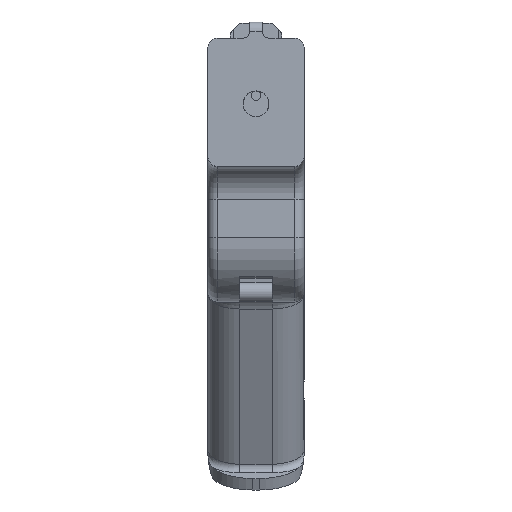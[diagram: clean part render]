
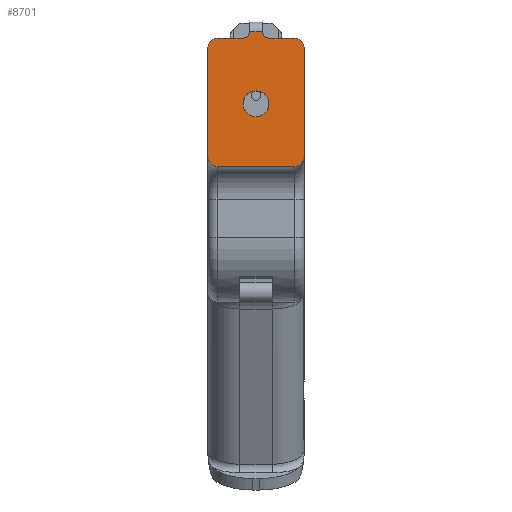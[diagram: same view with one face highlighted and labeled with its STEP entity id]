
A CAD part, top view. The second image highlights one B-rep face of the part: STEP entity #8701.
In plain terms, the highlighted planar face has unit normal (0, 0, 1).
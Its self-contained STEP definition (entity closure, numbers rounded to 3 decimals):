
#580=CARTESIAN_POINT('',(15.0,-3.,-20.));
#581=VERTEX_POINT('',#580);
#588=CARTESIAN_POINT('',(15.0,-37.,-20.));
#589=VERTEX_POINT('',#588);
#590=CARTESIAN_POINT('',(15.0,-3.,-20.));
#591=DIRECTION('',(0.0,-1.0,0.0));
#592=VECTOR('',#591,34.);
#593=LINE('',#590,#592);
#594=EDGE_CURVE('',#581,#589,#593,.T.);
#2318=CARTESIAN_POINT('',(-12.0,0.,-20.));
#2319=VERTEX_POINT('',#2318);
#2326=CARTESIAN_POINT('',(-4.0,0.,-20.));
#2327=VERTEX_POINT('',#2326);
#2328=CARTESIAN_POINT('',(-12.0,0.,-20.));
#2329=DIRECTION('',(1.0,0.0,0.0));
#2330=VECTOR('',#2329,8.0);
#2331=LINE('',#2328,#2330);
#2332=EDGE_CURVE('',#2319,#2327,#2331,.T.);
#2350=CARTESIAN_POINT('',(4.0,0.,-20.));
#2351=VERTEX_POINT('',#2350);
#2358=CARTESIAN_POINT('',(12.0,0.,-20.));
#2359=VERTEX_POINT('',#2358);
#2360=CARTESIAN_POINT('',(4.0,0.,-20.));
#2361=DIRECTION('',(1.0,0.0,0.0));
#2362=VECTOR('',#2361,8.0);
#2363=LINE('',#2360,#2362);
#2364=EDGE_CURVE('',#2351,#2359,#2363,.T.);
#8549=CARTESIAN_POINT('',(2.0,2.,-20.));
#8550=VERTEX_POINT('',#8549);
#8568=CARTESIAN_POINT('',(-2.0,2.,-20.));
#8569=VERTEX_POINT('',#8568);
#8577=CARTESIAN_POINT('',(-2.0,2.,-20.));
#8578=DIRECTION('',(1.0,0.0,0.0));
#8579=VECTOR('',#8578,4.0);
#8580=LINE('',#8577,#8579);
#8581=EDGE_CURVE('',#8569,#8550,#8580,.T.);
#8617=CARTESIAN_POINT('',(0.0,43.,-20.));
#8618=DIRECTION('',(0.0,0.0,-1.0));
#8619=DIRECTION('',(-1.0,0.0,0.0));
#8620=AXIS2_PLACEMENT_3D('',#8617,#8618,#8619);
#8621=PLANE('',#8620);
#8622=ORIENTED_EDGE('',*,*,#8581,.F.);
#8623=CARTESIAN_POINT('',(-4.0,2.,-20.));
#8624=DIRECTION('',(0.0,0.0,1.0));
#8625=DIRECTION('',(0.707,-0.707,0.0));
#8626=AXIS2_PLACEMENT_3D('',#8623,#8624,#8625);
#8627=CIRCLE('',#8626,2.0);
#8628=EDGE_CURVE('',#2327,#8569,#8627,.T.);
#8629=ORIENTED_EDGE('',*,*,#8628,.F.);
#8630=ORIENTED_EDGE('',*,*,#2332,.F.);
#8631=CARTESIAN_POINT('',(-15.0,-3.,-20.));
#8632=VERTEX_POINT('',#8631);
#8633=CARTESIAN_POINT('',(-12.0,-3.,-20.));
#8634=DIRECTION('',(0.0,0.0,-1.0));
#8635=DIRECTION('',(-0.707,0.707,0.0));
#8636=AXIS2_PLACEMENT_3D('',#8633,#8634,#8635);
#8637=CIRCLE('',#8636,3.);
#8638=EDGE_CURVE('',#8632,#2319,#8637,.T.);
#8639=ORIENTED_EDGE('',*,*,#8638,.F.);
#8640=CARTESIAN_POINT('',(-15.0,-37.,-20.));
#8641=VERTEX_POINT('',#8640);
#8642=CARTESIAN_POINT('',(-15.0,-37.,-20.));
#8643=DIRECTION('',(0.0,1.0,0.0));
#8644=VECTOR('',#8643,34.);
#8645=LINE('',#8642,#8644);
#8646=EDGE_CURVE('',#8641,#8632,#8645,.T.);
#8647=ORIENTED_EDGE('',*,*,#8646,.F.);
#8648=CARTESIAN_POINT('',(-12.0,-40.,-20.));
#8649=VERTEX_POINT('',#8648);
#8650=CARTESIAN_POINT('',(-12.0,-37.,-20.));
#8651=DIRECTION('',(0.0,0.0,-1.0));
#8652=DIRECTION('',(-0.707,-0.707,0.0));
#8653=AXIS2_PLACEMENT_3D('',#8650,#8651,#8652);
#8654=CIRCLE('',#8653,3.);
#8655=EDGE_CURVE('',#8649,#8641,#8654,.T.);
#8656=ORIENTED_EDGE('',*,*,#8655,.F.);
#8657=CARTESIAN_POINT('',(12.0,-40.,-20.));
#8658=VERTEX_POINT('',#8657);
#8659=CARTESIAN_POINT('',(12.0,-40.,-20.));
#8660=DIRECTION('',(-1.0,0.0,0.0));
#8661=VECTOR('',#8660,24.0);
#8662=LINE('',#8659,#8661);
#8663=EDGE_CURVE('',#8658,#8649,#8662,.T.);
#8664=ORIENTED_EDGE('',*,*,#8663,.F.);
#8665=CARTESIAN_POINT('',(12.0,-37.,-20.));
#8666=DIRECTION('',(0.0,0.0,-1.0));
#8667=DIRECTION('',(0.707,-0.707,0.0));
#8668=AXIS2_PLACEMENT_3D('',#8665,#8666,#8667);
#8669=CIRCLE('',#8668,3.);
#8670=EDGE_CURVE('',#589,#8658,#8669,.T.);
#8671=ORIENTED_EDGE('',*,*,#8670,.F.);
#8672=ORIENTED_EDGE('',*,*,#594,.F.);
#8673=CARTESIAN_POINT('',(12.0,-3.,-20.));
#8674=DIRECTION('',(0.0,0.0,-1.0));
#8675=DIRECTION('',(0.707,0.707,0.0));
#8676=AXIS2_PLACEMENT_3D('',#8673,#8674,#8675);
#8677=CIRCLE('',#8676,3.);
#8678=EDGE_CURVE('',#2359,#581,#8677,.T.);
#8679=ORIENTED_EDGE('',*,*,#8678,.F.);
#8680=ORIENTED_EDGE('',*,*,#2364,.F.);
#8681=CARTESIAN_POINT('',(4.0,2.,-20.));
#8682=DIRECTION('',(0.0,0.0,1.0));
#8683=DIRECTION('',(-0.707,-0.707,0.0));
#8684=AXIS2_PLACEMENT_3D('',#8681,#8682,#8683);
#8685=CIRCLE('',#8684,2.0);
#8686=EDGE_CURVE('',#8550,#2351,#8685,.T.);
#8687=ORIENTED_EDGE('',*,*,#8686,.F.);
#8688=EDGE_LOOP('',(#8622,#8629,#8630,#8639,#8647,#8656,#8664,#8671,#8672,#8679,#8680,#8687));
#8689=FACE_OUTER_BOUND('',#8688,.T.);
#8690=CARTESIAN_POINT('',(4.0,-20.5,-20.));
#8691=VERTEX_POINT('',#8690);
#8692=CARTESIAN_POINT('',(0.0,-20.5,-20.));
#8693=DIRECTION('',(0.0,0.0,1.0));
#8694=DIRECTION('',(-1.0,0.0,0.0));
#8695=AXIS2_PLACEMENT_3D('',#8692,#8693,#8694);
#8696=CIRCLE('',#8695,4.0);
#8697=EDGE_CURVE('',#8691,#8691,#8696,.T.);
#8698=ORIENTED_EDGE('',*,*,#8697,.F.);
#8699=EDGE_LOOP('',(#8698));
#8700=FACE_BOUND('',#8699,.T.);
#8701=ADVANCED_FACE('',(#8689,#8700),#8621,.F.);
